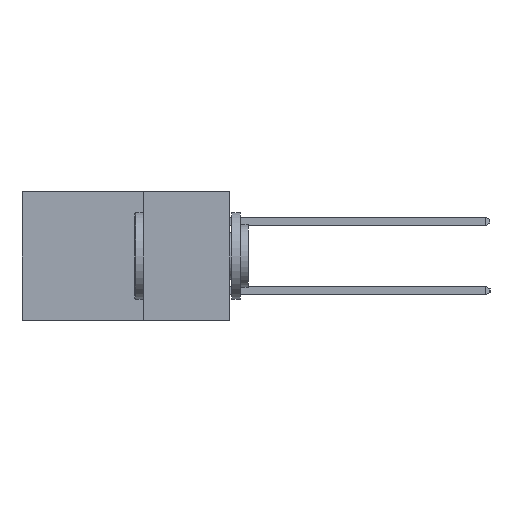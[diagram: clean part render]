
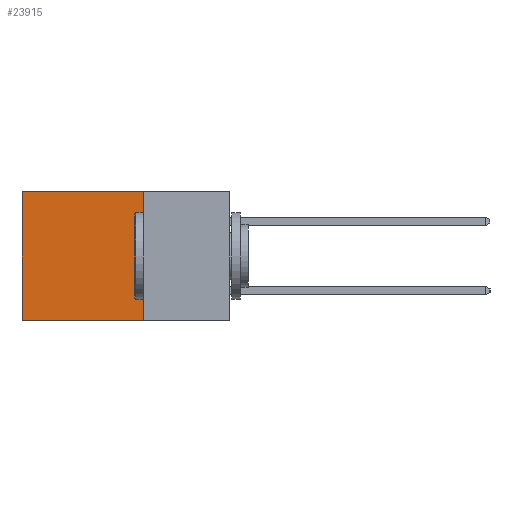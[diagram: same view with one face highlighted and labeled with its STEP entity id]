
A CAD part, left-side view. The second image highlights one B-rep face of the part: STEP entity #23915.
In plain terms, the highlighted planar face has unit normal (-1, 0, 0).
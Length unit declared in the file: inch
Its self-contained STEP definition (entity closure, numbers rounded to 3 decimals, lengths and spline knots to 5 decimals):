
#949 = VERTEX_POINT ( 'NONE', #2585 ) ;
#2585 = CARTESIAN_POINT ( 'NONE',  ( 0.2615, 0.6, 0. ) ) ;
#2839 = CARTESIAN_POINT ( 'NONE',  ( 0.2615, 0.25, 0. ) ) ;
#4050 = VERTEX_POINT ( 'NONE', #12959 ) ;
#4089 = VECTOR ( 'NONE', #21036, 39.37008 ) ;
#4501 = VERTEX_POINT ( 'NONE', #15718 ) ;
#4503 = CARTESIAN_POINT ( 'NONE',  ( 0.2615, 0.25, -0.37 ) ) ;
#4907 = DIRECTION ( 'NONE',  ( 0., 1., 0. ) ) ;
#4980 = EDGE_CURVE ( 'NONE', #23222, #4050, #15073, .T. ) ;
#6058 = VECTOR ( 'NONE', #11585, 39.37008 ) ;
#6612 = EDGE_CURVE ( 'NONE', #949, #4050, #6700, .T. ) ;
#6700 = LINE ( 'NONE', #19975, #6058 ) ;
#8139 = EDGE_CURVE ( 'NONE', #4501, #23222, #18916, .T. ) ;
#8494 = DIRECTION ( 'NONE',  ( 1., 0., 0. ) ) ;
#11310 = CARTESIAN_POINT ( 'NONE',  ( 0.2615, 0.25, -0.37 ) ) ;
#11585 = DIRECTION ( 'NONE',  ( 0., 0., -1. ) ) ;
#12155 = DIRECTION ( 'NONE',  ( 0., 0., -1. ) ) ;
#12959 = CARTESIAN_POINT ( 'NONE',  ( 0.2615, 0.6, -0.37 ) ) ;
#13414 = VECTOR ( 'NONE', #12155, 39.37008 ) ;
#14202 = VECTOR ( 'NONE', #4907, 39.37008 ) ;
#14595 = PLANE ( 'NONE',  #15390 ) ;
#14845 = LINE ( 'NONE', #2839, #14202 ) ;
#14895 = FACE_OUTER_BOUND ( 'NONE', #20920, .T. ) ;
#15073 = LINE ( 'NONE', #4503, #4089 ) ;
#15390 = AXIS2_PLACEMENT_3D ( 'NONE', #20835, #8494, #22897 ) ;
#15533 = ORIENTED_EDGE ( 'NONE', *, *, #8139, .F. ) ;
#15718 = CARTESIAN_POINT ( 'NONE',  ( 0.2615, 0.25, 0. ) ) ;
#16401 = ORIENTED_EDGE ( 'NONE', *, *, #4980, .F. ) ;
#18276 = CARTESIAN_POINT ( 'NONE',  ( 0.2615, 0.25, -0.37 ) ) ;
#18916 = LINE ( 'NONE', #18276, #13414 ) ;
#19975 = CARTESIAN_POINT ( 'NONE',  ( 0.2615, 0.6, -0.37 ) ) ;
#20835 = CARTESIAN_POINT ( 'NONE',  ( 0.2615, 0.25, -0.37 ) ) ;
#20920 = EDGE_LOOP ( 'NONE', ( #25782, #16401, #15533, #23400 ) ) ;
#21036 = DIRECTION ( 'NONE',  ( 0., 1., 0. ) ) ;
#22897 = DIRECTION ( 'NONE',  ( 0., 0., -1. ) ) ;
#23222 = VERTEX_POINT ( 'NONE', #11310 ) ;
#23400 = ORIENTED_EDGE ( 'NONE', *, *, #24614, .T. ) ;
#23915 = ADVANCED_FACE ( 'NONE', ( #14895 ), #14595, .F. ) ;
#24614 = EDGE_CURVE ( 'NONE', #4501, #949, #14845, .T. ) ;
#25782 = ORIENTED_EDGE ( 'NONE', *, *, #6612, .T. ) ;
